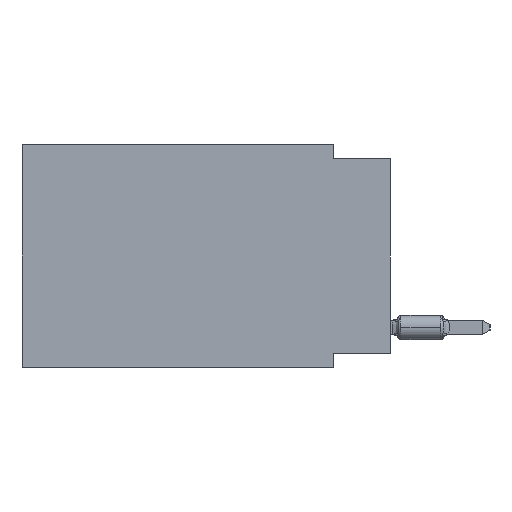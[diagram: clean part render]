
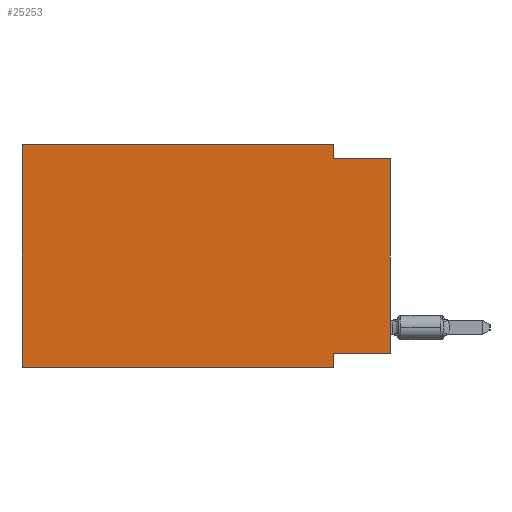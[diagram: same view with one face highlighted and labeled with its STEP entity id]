
A CAD part, left-side view. The second image highlights one B-rep face of the part: STEP entity #25253.
In plain terms, the highlighted planar face has unit normal (-1, 0, 0).
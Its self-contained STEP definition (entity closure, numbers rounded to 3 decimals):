
#2140 = EDGE_CURVE ( 'NONE', #28635, #29259, #15559, .T. ) ;
#2449 = LINE ( 'NONE', #11922, #8258 ) ;
#2555 = DIRECTION ( 'NONE',  ( 0., 0., -1. ) ) ;
#2796 = VERTEX_POINT ( 'NONE', #37416 ) ;
#3237 = CARTESIAN_POINT ( 'NONE',  ( 0., 0., -0.635 ) ) ;
#3272 = CARTESIAN_POINT ( 'NONE',  ( 0., 2.54, -0.635 ) ) ;
#3770 = CARTESIAN_POINT ( 'NONE',  ( 0., 16.383, 0. ) ) ;
#4554 = VECTOR ( 'NONE', #31522, 1000. ) ;
#5726 = DIRECTION ( 'NONE',  ( 0., -1., 0. ) ) ;
#6718 = ORIENTED_EDGE ( 'NONE', *, *, #2140, .T. ) ;
#7375 = ORIENTED_EDGE ( 'NONE', *, *, #39352, .F. ) ;
#7566 = VECTOR ( 'NONE', #2555, 1000. ) ;
#8258 = VECTOR ( 'NONE', #14649, 1000. ) ;
#9263 = CARTESIAN_POINT ( 'NONE',  ( 0., 16.383, -9.906 ) ) ;
#9350 = ORIENTED_EDGE ( 'NONE', *, *, #17995, .F. ) ;
#10004 = DIRECTION ( 'NONE',  ( 0., 1., 0. ) ) ;
#10560 = EDGE_CURVE ( 'NONE', #23358, #2796, #28652, .T. ) ;
#11795 = DIRECTION ( 'NONE',  ( 0., 0., 1. ) ) ;
#11922 = CARTESIAN_POINT ( 'NONE',  ( 0., 0., -0.635 ) ) ;
#12905 = EDGE_CURVE ( 'NONE', #23358, #18381, #33083, .T. ) ;
#13210 = CARTESIAN_POINT ( 'NONE',  ( 0., 2.54, 0. ) ) ;
#13755 = AXIS2_PLACEMENT_3D ( 'NONE', #34285, #30526, #14341 ) ;
#14049 = EDGE_CURVE ( 'NONE', #28635, #14192, #16502, .T. ) ;
#14192 = VERTEX_POINT ( 'NONE', #33087 ) ;
#14341 = DIRECTION ( 'NONE',  ( 0., 0., -1. ) ) ;
#14361 = CARTESIAN_POINT ( 'NONE',  ( 0., 2.54, -9.906 ) ) ;
#14649 = DIRECTION ( 'NONE',  ( 0., -1., 0. ) ) ;
#14903 = CARTESIAN_POINT ( 'NONE',  ( 0., 2.54, 0. ) ) ;
#14967 = FACE_OUTER_BOUND ( 'NONE', #22123, .T. ) ;
#14986 = LINE ( 'NONE', #14361, #27806 ) ;
#15559 = LINE ( 'NONE', #40575, #30976 ) ;
#16419 = ORIENTED_EDGE ( 'NONE', *, *, #10560, .T. ) ;
#16502 = LINE ( 'NONE', #22817, #23547 ) ;
#17903 = PLANE ( 'NONE',  #13755 ) ;
#17995 = EDGE_CURVE ( 'NONE', #14192, #2796, #14986, .T. ) ;
#18381 = VERTEX_POINT ( 'NONE', #3770 ) ;
#19001 = ORIENTED_EDGE ( 'NONE', *, *, #14049, .F. ) ;
#22123 = EDGE_LOOP ( 'NONE', ( #6718, #7375, #34905, #22571, #38954, #16419, #9350, #19001 ) ) ;
#22571 = ORIENTED_EDGE ( 'NONE', *, *, #28498, .F. ) ;
#22817 = CARTESIAN_POINT ( 'NONE',  ( 0., 0., -9.271 ) ) ;
#23358 = VERTEX_POINT ( 'NONE', #30887 ) ;
#23547 = VECTOR ( 'NONE', #10004, 1000. ) ;
#25253 = ADVANCED_FACE ( 'NONE', ( #14967 ), #17903, .F. ) ;
#26022 = VECTOR ( 'NONE', #5726, 1000. ) ;
#27196 = DIRECTION ( 'NONE',  ( 0., 0., -1. ) ) ;
#27806 = VECTOR ( 'NONE', #27196, 1000. ) ;
#28498 = EDGE_CURVE ( 'NONE', #18381, #36337, #31760, .T. ) ;
#28635 = VERTEX_POINT ( 'NONE', #35330 ) ;
#28652 = LINE ( 'NONE', #9263, #4554 ) ;
#29191 = LINE ( 'NONE', #13210, #7566 ) ;
#29259 = VERTEX_POINT ( 'NONE', #3237 ) ;
#29525 = VECTOR ( 'NONE', #39790, 1000. ) ;
#30526 = DIRECTION ( 'NONE',  ( 1., 0., 0. ) ) ;
#30887 = CARTESIAN_POINT ( 'NONE',  ( 0., 16.383, -9.906 ) ) ;
#30976 = VECTOR ( 'NONE', #11795, 1000. ) ;
#31522 = DIRECTION ( 'NONE',  ( 0., -1., 0. ) ) ;
#31760 = LINE ( 'NONE', #38071, #26022 ) ;
#33083 = LINE ( 'NONE', #36034, #29525 ) ;
#33087 = CARTESIAN_POINT ( 'NONE',  ( 0., 2.54, -9.271 ) ) ;
#34285 = CARTESIAN_POINT ( 'NONE',  ( 0., 16.383, 0. ) ) ;
#34905 = ORIENTED_EDGE ( 'NONE', *, *, #39087, .F. ) ;
#35330 = CARTESIAN_POINT ( 'NONE',  ( 0., 0., -9.271 ) ) ;
#36034 = CARTESIAN_POINT ( 'NONE',  ( 0., 16.383, 0. ) ) ;
#36337 = VERTEX_POINT ( 'NONE', #14903 ) ;
#37416 = CARTESIAN_POINT ( 'NONE',  ( 0., 2.54, -9.906 ) ) ;
#38071 = CARTESIAN_POINT ( 'NONE',  ( 0., 16.383, 0. ) ) ;
#38329 = VERTEX_POINT ( 'NONE', #3272 ) ;
#38954 = ORIENTED_EDGE ( 'NONE', *, *, #12905, .F. ) ;
#39087 = EDGE_CURVE ( 'NONE', #36337, #38329, #29191, .T. ) ;
#39352 = EDGE_CURVE ( 'NONE', #38329, #29259, #2449, .T. ) ;
#39790 = DIRECTION ( 'NONE',  ( 0., 0., 1. ) ) ;
#40575 = CARTESIAN_POINT ( 'NONE',  ( 0., 0., 0. ) ) ;
